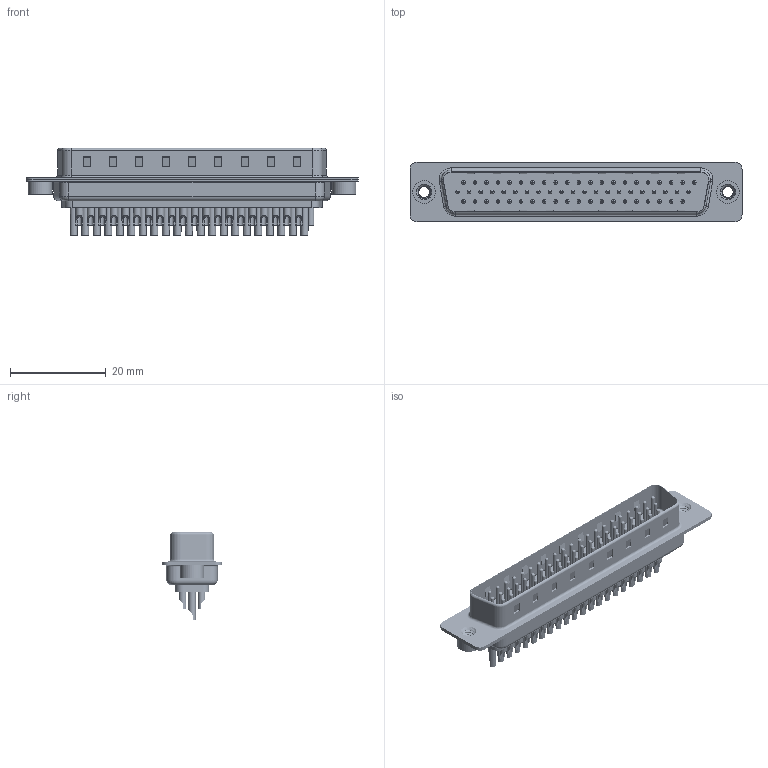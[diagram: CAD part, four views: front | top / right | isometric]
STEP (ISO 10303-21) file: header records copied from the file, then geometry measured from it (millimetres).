
FILE_DESCRIPTION (( 'STEP AP203' ), '1' );
FILE_NAME ('637-M62-632-BT2.STEP', '2018-11-20T03:23:40', ( '' ), ( '' ), 'SwSTEP 2.0', 'SolidWorks 2016', '' );
FILE_SCHEMA (( 'CONFIG_CONTROL_DESIGN' ));
Length unit declared in the file: millimetre
Products named in the file (8): 637M 4-40 Threaded Rivet; 637-M62-632-BT2; 637M Housing_62 Contacts; 637M Shell Front_62 Contacts; 637M Shell Rear_62 Contacts; 637M Contact Row 1_32; 637M Contact Row 2_32; 637M Contact Row 3_32
Assembly tree (67 placements, depth 2):
  637-M62-632-BT2
    637M Housing_62 Contacts
    637M Shell Front_62 Contacts
    637M Shell Rear_62 Contacts
    637M Contact Row 1_32  x21
    637M Contact Row 2_32  x21
    637M Contact Row 3_32  x20
    637M 4-40 Threaded Rivet  x2
Bounding box: 69.4 x 12.5 x 18.25 mm (x, y, z)
Volume: 4122.4 mm3; surface area: 12177.1 mm2
Topology: 67 solids, 67 shells, 2706 faces, 6265 edges, 3828 vertices
Faces by surface type: cylinder 1133, plane 761, torus 670, cone 136, bspline 6
Entity records: 32656 total; most frequent: CARTESIAN_POINT 6434, DIRECTION 5408, ORIENTED_EDGE 4568, EDGE_CURVE 2284, AXIS2_PLACEMENT_3D 2172, VERTEX_POINT 1475, EDGE_LOOP 1275, CIRCLE 1143
